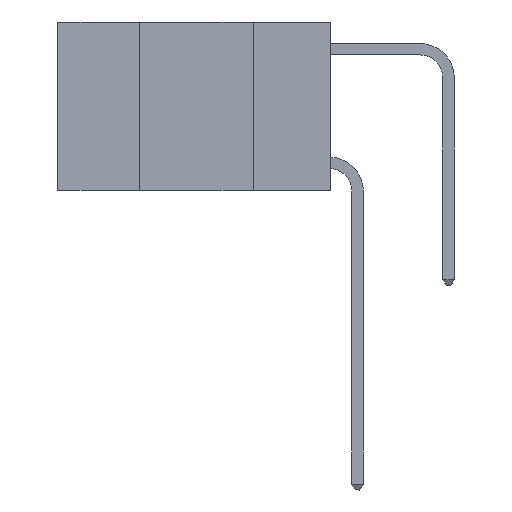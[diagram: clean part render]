
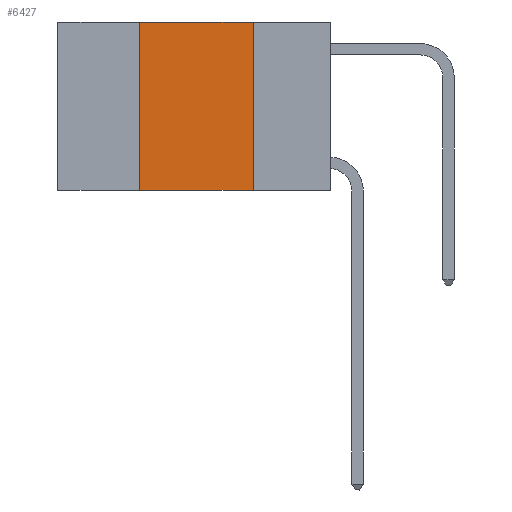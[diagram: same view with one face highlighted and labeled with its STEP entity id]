
A CAD part, left-side view. The second image highlights one B-rep face of the part: STEP entity #6427.
In plain terms, the highlighted planar face has unit normal (-1, 0, 0).
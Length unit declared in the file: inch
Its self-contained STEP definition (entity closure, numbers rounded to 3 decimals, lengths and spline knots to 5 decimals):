
#790 = EDGE_CURVE ( 'NONE', #3674, #8591, #7676, .T. ) ;
#854 = ORIENTED_EDGE ( 'NONE', *, *, #7734, .F. ) ;
#1010 = DIRECTION ( 'NONE',  ( 0., 0., -1. ) ) ;
#1213 = AXIS2_PLACEMENT_3D ( 'NONE', #3139, #6273, #1651 ) ;
#1616 = ORIENTED_EDGE ( 'NONE', *, *, #790, .F. ) ;
#1651 = DIRECTION ( 'NONE',  ( 0., 0., -1. ) ) ;
#2051 = EDGE_LOOP ( 'NONE', ( #854, #1616, #9197, #3433 ) ) ;
#2169 = VECTOR ( 'NONE', #10154, 39.37008 ) ;
#3139 = CARTESIAN_POINT ( 'NONE',  ( 0., 0.6, 0. ) ) ;
#3252 = EDGE_CURVE ( 'NONE', #3826, #3674, #6228, .T. ) ;
#3433 = ORIENTED_EDGE ( 'NONE', *, *, #4423, .T. ) ;
#3545 = CARTESIAN_POINT ( 'NONE',  ( 0., 0.42, -0.37 ) ) ;
#3674 = VERTEX_POINT ( 'NONE', #8739 ) ;
#3826 = VERTEX_POINT ( 'NONE', #3545 ) ;
#4120 = CARTESIAN_POINT ( 'NONE',  ( 0., 0.17, 0. ) ) ;
#4123 = VERTEX_POINT ( 'NONE', #9093 ) ;
#4423 = EDGE_CURVE ( 'NONE', #3826, #4123, #5992, .T. ) ;
#4622 = CARTESIAN_POINT ( 'NONE',  ( 0., 0.6, -0.37 ) ) ;
#4905 = LINE ( 'NONE', #7245, #8636 ) ;
#5992 = LINE ( 'NONE', #4622, #2169 ) ;
#6228 = LINE ( 'NONE', #9679, #6358 ) ;
#6273 = DIRECTION ( 'NONE',  ( 1., 0., 0. ) ) ;
#6358 = VECTOR ( 'NONE', #6592, 39.37008 ) ;
#6427 = ADVANCED_FACE ( 'NONE', ( #7839 ), #7936, .F. ) ;
#6592 = DIRECTION ( 'NONE',  ( 0., 0., 1. ) ) ;
#6802 = DIRECTION ( 'NONE',  ( 0., -1., 0. ) ) ;
#7245 = CARTESIAN_POINT ( 'NONE',  ( 0., 0.17, 0. ) ) ;
#7410 = VECTOR ( 'NONE', #6802, 39.37008 ) ;
#7676 = LINE ( 'NONE', #8449, #7410 ) ;
#7734 = EDGE_CURVE ( 'NONE', #8591, #4123, #4905, .T. ) ;
#7839 = FACE_OUTER_BOUND ( 'NONE', #2051, .T. ) ;
#7936 = PLANE ( 'NONE',  #1213 ) ;
#8449 = CARTESIAN_POINT ( 'NONE',  ( 0., 0.6, 0. ) ) ;
#8591 = VERTEX_POINT ( 'NONE', #4120 ) ;
#8636 = VECTOR ( 'NONE', #1010, 39.37008 ) ;
#8739 = CARTESIAN_POINT ( 'NONE',  ( 0., 0.42, 0. ) ) ;
#9093 = CARTESIAN_POINT ( 'NONE',  ( 0., 0.17, -0.37 ) ) ;
#9197 = ORIENTED_EDGE ( 'NONE', *, *, #3252, .F. ) ;
#9679 = CARTESIAN_POINT ( 'NONE',  ( 0., 0.42, 0. ) ) ;
#10154 = DIRECTION ( 'NONE',  ( 0., -1., 0. ) ) ;
